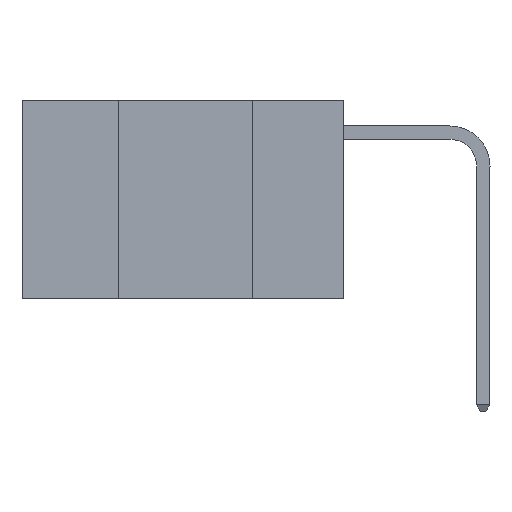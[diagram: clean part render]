
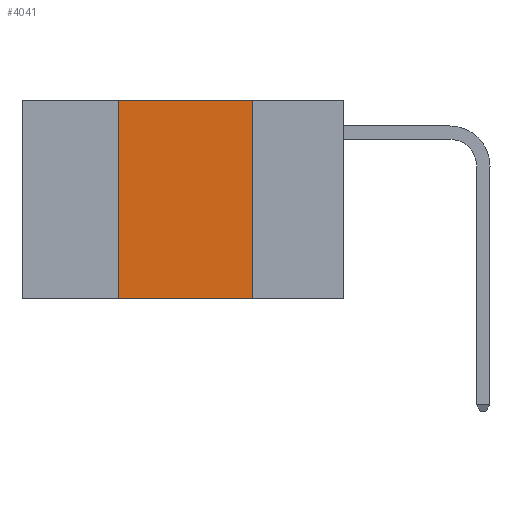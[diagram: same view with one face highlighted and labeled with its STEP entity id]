
A CAD part, left-side view. The second image highlights one B-rep face of the part: STEP entity #4041.
In plain terms, the highlighted planar face has unit normal (-1, 0, 0).
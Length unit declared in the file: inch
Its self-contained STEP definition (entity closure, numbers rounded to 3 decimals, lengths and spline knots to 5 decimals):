
#265 = EDGE_CURVE ( 'NONE', #7112, #9241, #12013, .T. ) ;
#269 = EDGE_CURVE ( 'NONE', #7112, #5689, #6724, .T. ) ;
#333 = EDGE_CURVE ( 'NONE', #7812, #9241, #10853, .T. ) ;
#478 = CARTESIAN_POINT ( 'NONE',  ( 0., 0.42, 0. ) ) ;
#627 = AXIS2_PLACEMENT_3D ( 'NONE', #2859, #3966, #11326 ) ;
#1076 = ORIENTED_EDGE ( 'NONE', *, *, #333, .F. ) ;
#1323 = CARTESIAN_POINT ( 'NONE',  ( 0., 0.17, 0. ) ) ;
#2313 = VECTOR ( 'NONE', #7884, 39.37008 ) ;
#2859 = CARTESIAN_POINT ( 'NONE',  ( 0., 0.6, 0. ) ) ;
#2905 = CARTESIAN_POINT ( 'NONE',  ( 0., 0.42, -0.37 ) ) ;
#3687 = VECTOR ( 'NONE', #4553, 39.37008 ) ;
#3966 = DIRECTION ( 'NONE',  ( 1., 0., 0. ) ) ;
#4041 = ADVANCED_FACE ( 'NONE', ( #7953 ), #8352, .F. ) ;
#4553 = DIRECTION ( 'NONE',  ( 0., -1., 0. ) ) ;
#4809 = DIRECTION ( 'NONE',  ( 0., 0., 1. ) ) ;
#5176 = EDGE_CURVE ( 'NONE', #5689, #7812, #5567, .T. ) ;
#5567 = LINE ( 'NONE', #12502, #11303 ) ;
#5689 = VERTEX_POINT ( 'NONE', #11961 ) ;
#6515 = DIRECTION ( 'NONE',  ( 0., -1., 0. ) ) ;
#6724 = LINE ( 'NONE', #478, #11719 ) ;
#6734 = ORIENTED_EDGE ( 'NONE', *, *, #265, .T. ) ;
#7112 = VERTEX_POINT ( 'NONE', #2905 ) ;
#7812 = VERTEX_POINT ( 'NONE', #10301 ) ;
#7884 = DIRECTION ( 'NONE',  ( 0., 0., -1. ) ) ;
#7953 = FACE_OUTER_BOUND ( 'NONE', #8252, .T. ) ;
#8211 = ORIENTED_EDGE ( 'NONE', *, *, #269, .F. ) ;
#8252 = EDGE_LOOP ( 'NONE', ( #1076, #13591, #8211, #6734 ) ) ;
#8352 = PLANE ( 'NONE',  #627 ) ;
#9241 = VERTEX_POINT ( 'NONE', #11117 ) ;
#10301 = CARTESIAN_POINT ( 'NONE',  ( 0., 0.17, 0. ) ) ;
#10853 = LINE ( 'NONE', #1323, #2313 ) ;
#11058 = CARTESIAN_POINT ( 'NONE',  ( 0., 0.6, -0.37 ) ) ;
#11117 = CARTESIAN_POINT ( 'NONE',  ( 0., 0.17, -0.37 ) ) ;
#11303 = VECTOR ( 'NONE', #6515, 39.37008 ) ;
#11326 = DIRECTION ( 'NONE',  ( 0., 0., -1. ) ) ;
#11719 = VECTOR ( 'NONE', #4809, 39.37008 ) ;
#11961 = CARTESIAN_POINT ( 'NONE',  ( 0., 0.42, 0. ) ) ;
#12013 = LINE ( 'NONE', #11058, #3687 ) ;
#12502 = CARTESIAN_POINT ( 'NONE',  ( 0., 0.6, 0. ) ) ;
#13591 = ORIENTED_EDGE ( 'NONE', *, *, #5176, .F. ) ;
